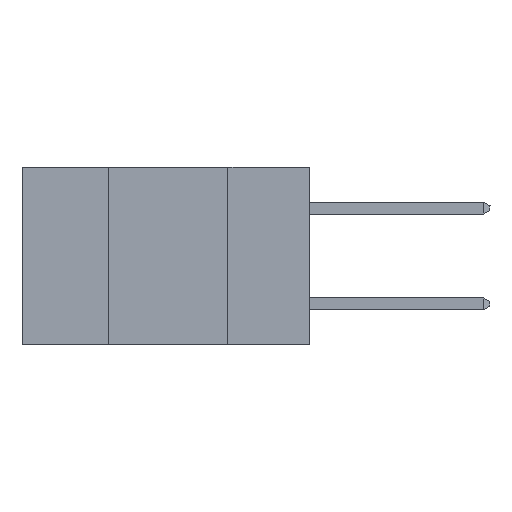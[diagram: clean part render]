
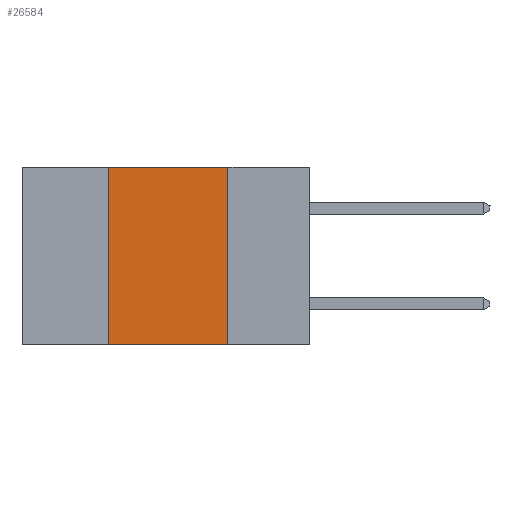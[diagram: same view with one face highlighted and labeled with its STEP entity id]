
A CAD part, left-side view. The second image highlights one B-rep face of the part: STEP entity #26584.
In plain terms, the highlighted planar face has unit normal (-1, 0, 0).
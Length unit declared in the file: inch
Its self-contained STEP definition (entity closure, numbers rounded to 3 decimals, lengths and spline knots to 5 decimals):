
#57 = DIRECTION ( 'NONE',  ( 0., -1., 0. ) ) ;
#657 = CARTESIAN_POINT ( 'NONE',  ( 0., 0.17, 0. ) ) ;
#903 = CARTESIAN_POINT ( 'NONE',  ( 0., 0.6, 0. ) ) ;
#1845 = LINE ( 'NONE', #18856, #32841 ) ;
#3122 = EDGE_CURVE ( 'NONE', #23291, #11743, #19505, .T. ) ;
#5939 = VERTEX_POINT ( 'NONE', #34546 ) ;
#6854 = VECTOR ( 'NONE', #13867, 39.37008 ) ;
#10415 = PLANE ( 'NONE',  #33834 ) ;
#11532 = FACE_OUTER_BOUND ( 'NONE', #21014, .T. ) ;
#11553 = ORIENTED_EDGE ( 'NONE', *, *, #17129, .F. ) ;
#11743 = VERTEX_POINT ( 'NONE', #34919 ) ;
#12235 = VERTEX_POINT ( 'NONE', #657 ) ;
#13539 = DIRECTION ( 'NONE',  ( 1., 0., 0. ) ) ;
#13867 = DIRECTION ( 'NONE',  ( 0., 0., 1. ) ) ;
#15234 = VECTOR ( 'NONE', #57, 39.37008 ) ;
#15439 = ORIENTED_EDGE ( 'NONE', *, *, #19127, .F. ) ;
#16615 = DIRECTION ( 'NONE',  ( 0., 0., -1. ) ) ;
#17129 = EDGE_CURVE ( 'NONE', #23291, #5939, #28665, .T. ) ;
#18413 = DIRECTION ( 'NONE',  ( 0., -1., 0. ) ) ;
#18856 = CARTESIAN_POINT ( 'NONE',  ( 0., 0.17, 0. ) ) ;
#18992 = CARTESIAN_POINT ( 'NONE',  ( 0., 0.42, -0.37 ) ) ;
#19127 = EDGE_CURVE ( 'NONE', #12235, #11743, #1845, .T. ) ;
#19505 = LINE ( 'NONE', #31067, #28683 ) ;
#21014 = EDGE_LOOP ( 'NONE', ( #15439, #23466, #11553, #30309 ) ) ;
#22237 = DIRECTION ( 'NONE',  ( 0., 0., -1. ) ) ;
#23291 = VERTEX_POINT ( 'NONE', #18992 ) ;
#23466 = ORIENTED_EDGE ( 'NONE', *, *, #38975, .F. ) ;
#26584 = ADVANCED_FACE ( 'NONE', ( #11532 ), #10415, .F. ) ;
#27828 = LINE ( 'NONE', #39647, #15234 ) ;
#28665 = LINE ( 'NONE', #32768, #6854 ) ;
#28683 = VECTOR ( 'NONE', #18413, 39.37008 ) ;
#30309 = ORIENTED_EDGE ( 'NONE', *, *, #3122, .T. ) ;
#31067 = CARTESIAN_POINT ( 'NONE',  ( 0., 0.6, -0.37 ) ) ;
#32768 = CARTESIAN_POINT ( 'NONE',  ( 0., 0.42, 0. ) ) ;
#32841 = VECTOR ( 'NONE', #22237, 39.37008 ) ;
#33834 = AXIS2_PLACEMENT_3D ( 'NONE', #903, #13539, #16615 ) ;
#34546 = CARTESIAN_POINT ( 'NONE',  ( 0., 0.42, 0. ) ) ;
#34919 = CARTESIAN_POINT ( 'NONE',  ( 0., 0.17, -0.37 ) ) ;
#38975 = EDGE_CURVE ( 'NONE', #5939, #12235, #27828, .T. ) ;
#39647 = CARTESIAN_POINT ( 'NONE',  ( 0., 0.6, 0. ) ) ;
